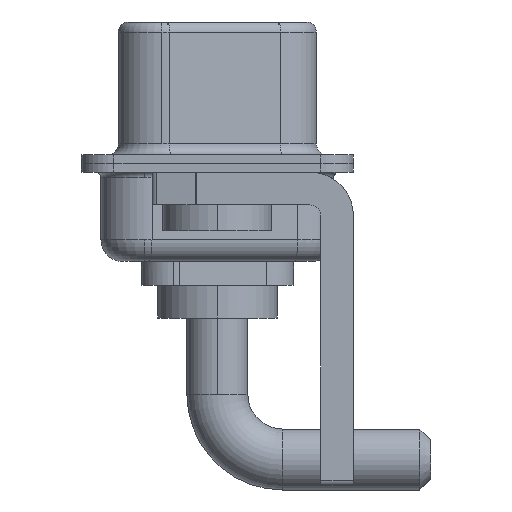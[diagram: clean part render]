
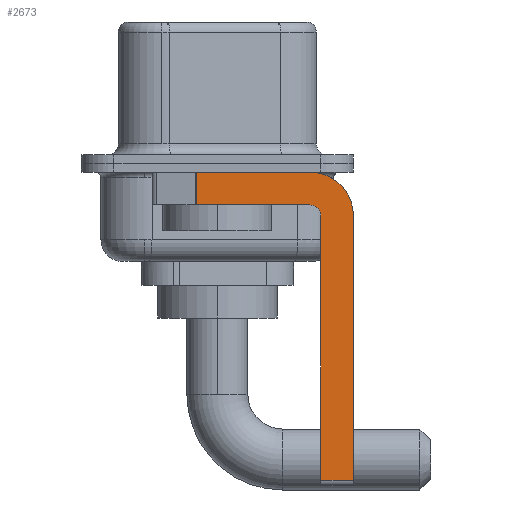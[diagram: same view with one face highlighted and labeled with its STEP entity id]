
A CAD part, left-side view. The second image highlights one B-rep face of the part: STEP entity #2673.
In plain terms, the highlighted planar face has unit normal (-1, 0, 0).
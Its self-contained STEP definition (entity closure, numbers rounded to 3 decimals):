
#65 = PLANE ( 'NONE',  #254 ) ;
#67 = VECTOR ( 'NONE', #15458, 1000. ) ;
#70 = EDGE_CURVE ( 'NONE', #15096, #10602, #4154, .T. ) ;
#207 = VECTOR ( 'NONE', #13800, 1000. ) ;
#254 = AXIS2_PLACEMENT_3D ( 'NONE', #4029, #6786, #2895 ) ;
#288 = AXIS2_PLACEMENT_3D ( 'NONE', #10589, #9136, #2586 ) ;
#394 = ORIENTED_EDGE ( 'NONE', *, *, #14246, .T. ) ;
#583 = CARTESIAN_POINT ( 'NONE',  ( -2.9, -6.25, -2.4 ) ) ;
#635 = VERTEX_POINT ( 'NONE', #11191 ) ;
#715 = VERTEX_POINT ( 'NONE', #7983 ) ;
#857 = CARTESIAN_POINT ( 'NONE',  ( -2.9, -4.75, -14.8 ) ) ;
#1333 = AXIS2_PLACEMENT_3D ( 'NONE', #9251, #15636, #10374 ) ;
#1522 = FACE_OUTER_BOUND ( 'NONE', #6652, .T. ) ;
#1954 = CARTESIAN_POINT ( 'NONE',  ( -2.9, -6.25, -2.4 ) ) ;
#2011 = DIRECTION ( 'NONE',  ( 0., -1., 0. ) ) ;
#2586 = DIRECTION ( 'NONE',  ( 0., 0., -1. ) ) ;
#2673 = ADVANCED_FACE ( 'NONE', ( #1522 ), #65, .F. ) ;
#2895 = DIRECTION ( 'NONE',  ( 0., 0., -1. ) ) ;
#2932 = DIRECTION ( 'NONE',  ( 0., 1., 0. ) ) ;
#4029 = CARTESIAN_POINT ( 'NONE',  ( -2.9, -4.25, -2.4 ) ) ;
#4154 = CIRCLE ( 'NONE', #288, 2. ) ;
#4371 = CARTESIAN_POINT ( 'NONE',  ( -2.9, 0.978, -1.9 ) ) ;
#4441 = CARTESIAN_POINT ( 'NONE',  ( -2.9, -6.25, -14.55 ) ) ;
#4662 = VERTEX_POINT ( 'NONE', #11510 ) ;
#5641 = LINE ( 'NONE', #10891, #13351 ) ;
#5760 = ORIENTED_EDGE ( 'NONE', *, *, #15712, .F. ) ;
#6184 = VECTOR ( 'NONE', #16093, 1000. ) ;
#6215 = EDGE_CURVE ( 'NONE', #10602, #13863, #10454, .T. ) ;
#6509 = LINE ( 'NONE', #8104, #12809 ) ;
#6652 = EDGE_LOOP ( 'NONE', ( #15838, #9174, #13905, #14070, #5760, #394, #12259, #10948 ) ) ;
#6786 = DIRECTION ( 'NONE',  ( 1., 0., 0. ) ) ;
#7186 = LINE ( 'NONE', #14861, #15596 ) ;
#7548 = CARTESIAN_POINT ( 'NONE',  ( -2.9, 0.978, -1.9 ) ) ;
#7699 = VERTEX_POINT ( 'NONE', #7548 ) ;
#7983 = CARTESIAN_POINT ( 'NONE',  ( -2.9, -4.25, -1.9 ) ) ;
#8104 = CARTESIAN_POINT ( 'NONE',  ( -2.9, -4.25, -1.9 ) ) ;
#8357 = CARTESIAN_POINT ( 'NONE',  ( -2.9, -4.75, -2.4 ) ) ;
#8532 = LINE ( 'NONE', #857, #207 ) ;
#8766 = CIRCLE ( 'NONE', #1333, 0.5 ) ;
#9136 = DIRECTION ( 'NONE',  ( 1., 0., 0. ) ) ;
#9174 = ORIENTED_EDGE ( 'NONE', *, *, #10684, .T. ) ;
#9251 = CARTESIAN_POINT ( 'NONE',  ( -2.9, -4.25, -2.4 ) ) ;
#10241 = VERTEX_POINT ( 'NONE', #8357 ) ;
#10374 = DIRECTION ( 'NONE',  ( 0., 0., 1. ) ) ;
#10454 = LINE ( 'NONE', #1954, #67 ) ;
#10589 = CARTESIAN_POINT ( 'NONE',  ( -2.9, -4.25, -2.4 ) ) ;
#10602 = VERTEX_POINT ( 'NONE', #583 ) ;
#10684 = EDGE_CURVE ( 'NONE', #635, #7699, #12129, .T. ) ;
#10891 = CARTESIAN_POINT ( 'NONE',  ( -2.9, 3., -0.4 ) ) ;
#10948 = ORIENTED_EDGE ( 'NONE', *, *, #70, .F. ) ;
#11191 = CARTESIAN_POINT ( 'NONE',  ( -2.9, 0.978, -0.4 ) ) ;
#11510 = CARTESIAN_POINT ( 'NONE',  ( -2.9, -4.75, -14.55 ) ) ;
#12129 = LINE ( 'NONE', #4371, #6184 ) ;
#12259 = ORIENTED_EDGE ( 'NONE', *, *, #6215, .F. ) ;
#12360 = EDGE_CURVE ( 'NONE', #635, #15096, #5641, .T. ) ;
#12703 = EDGE_CURVE ( 'NONE', #715, #7699, #6509, .T. ) ;
#12809 = VECTOR ( 'NONE', #2932, 1000. ) ;
#13351 = VECTOR ( 'NONE', #14876, 1000. ) ;
#13800 = DIRECTION ( 'NONE',  ( 0., 0., 1. ) ) ;
#13863 = VERTEX_POINT ( 'NONE', #4441 ) ;
#13905 = ORIENTED_EDGE ( 'NONE', *, *, #12703, .F. ) ;
#14070 = ORIENTED_EDGE ( 'NONE', *, *, #16180, .F. ) ;
#14246 = EDGE_CURVE ( 'NONE', #4662, #13863, #7186, .T. ) ;
#14861 = CARTESIAN_POINT ( 'NONE',  ( -2.9, -4.25, -14.55 ) ) ;
#14876 = DIRECTION ( 'NONE',  ( 0., -1., 0. ) ) ;
#15096 = VERTEX_POINT ( 'NONE', #16264 ) ;
#15458 = DIRECTION ( 'NONE',  ( 0., 0., -1. ) ) ;
#15596 = VECTOR ( 'NONE', #2011, 1000. ) ;
#15636 = DIRECTION ( 'NONE',  ( -1., 0., 0. ) ) ;
#15712 = EDGE_CURVE ( 'NONE', #4662, #10241, #8532, .T. ) ;
#15838 = ORIENTED_EDGE ( 'NONE', *, *, #12360, .F. ) ;
#16093 = DIRECTION ( 'NONE',  ( 0., 0., -1. ) ) ;
#16180 = EDGE_CURVE ( 'NONE', #10241, #715, #8766, .T. ) ;
#16264 = CARTESIAN_POINT ( 'NONE',  ( -2.9, -4.25, -0.4 ) ) ;
